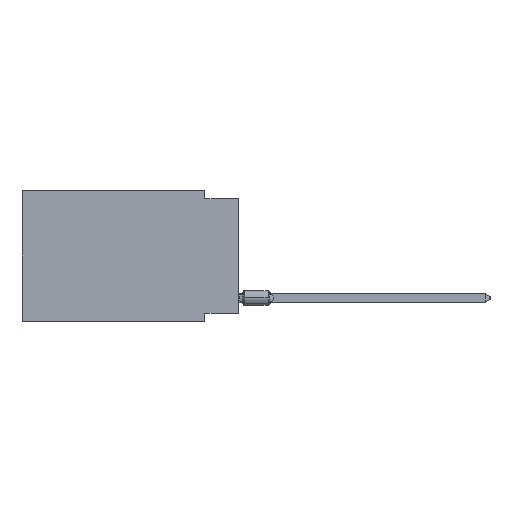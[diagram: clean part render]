
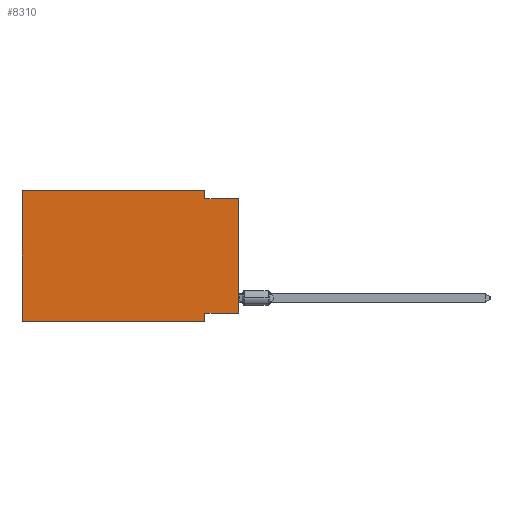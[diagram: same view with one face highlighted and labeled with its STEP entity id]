
A CAD part, left-side view. The second image highlights one B-rep face of the part: STEP entity #8310.
In plain terms, the highlighted planar face has unit normal (-1, 0, 0).
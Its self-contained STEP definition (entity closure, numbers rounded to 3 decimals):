
#1248 = VERTEX_POINT ( 'NONE', #43482 ) ;
#1774 = CARTESIAN_POINT ( 'NONE',  ( 0., 2.54, -9.906 ) ) ;
#2339 = ORIENTED_EDGE ( 'NONE', *, *, #16245, .F. ) ;
#3363 = EDGE_CURVE ( 'NONE', #26355, #38765, #23851, .T. ) ;
#3479 = VECTOR ( 'NONE', #33038, 1000. ) ;
#4649 = CARTESIAN_POINT ( 'NONE',  ( 0., 16.383, 0. ) ) ;
#5287 = EDGE_CURVE ( 'NONE', #26355, #52239, #14087, .T. ) ;
#5362 = AXIS2_PLACEMENT_3D ( 'NONE', #9798, #10987, #5902 ) ;
#5902 = DIRECTION ( 'NONE',  ( 0., 0., -1. ) ) ;
#6004 = VERTEX_POINT ( 'NONE', #13868 ) ;
#6097 = ORIENTED_EDGE ( 'NONE', *, *, #58985, .F. ) ;
#7154 = EDGE_CURVE ( 'NONE', #30819, #1248, #32797, .T. ) ;
#8310 = ADVANCED_FACE ( 'NONE', ( #32629 ), #10387, .F. ) ;
#9240 = VERTEX_POINT ( 'NONE', #26784 ) ;
#9586 = ORIENTED_EDGE ( 'NONE', *, *, #5287, .T. ) ;
#9798 = CARTESIAN_POINT ( 'NONE',  ( 0., 16.383, 0. ) ) ;
#10387 = PLANE ( 'NONE',  #5362 ) ;
#10987 = DIRECTION ( 'NONE',  ( 1., 0., 0. ) ) ;
#11818 = DIRECTION ( 'NONE',  ( 0., 1., 0. ) ) ;
#13607 = VECTOR ( 'NONE', #55955, 1000. ) ;
#13868 = CARTESIAN_POINT ( 'NONE',  ( 0., 2.54, 0. ) ) ;
#14087 = LINE ( 'NONE', #14392, #50177 ) ;
#14392 = CARTESIAN_POINT ( 'NONE',  ( 0., 16.383, -9.906 ) ) ;
#15633 = LINE ( 'NONE', #28853, #33295 ) ;
#16245 = EDGE_CURVE ( 'NONE', #48745, #52239, #25973, .T. ) ;
#20463 = VECTOR ( 'NONE', #31379, 1000. ) ;
#20588 = DIRECTION ( 'NONE',  ( 0., 0., -1. ) ) ;
#21037 = EDGE_CURVE ( 'NONE', #38765, #6004, #27648, .T. ) ;
#22013 = LINE ( 'NONE', #44787, #28293 ) ;
#22168 = CARTESIAN_POINT ( 'NONE',  ( 0., 0., -9.271 ) ) ;
#23208 = VECTOR ( 'NONE', #20588, 1000. ) ;
#23851 = LINE ( 'NONE', #4649, #13607 ) ;
#25973 = LINE ( 'NONE', #34981, #23208 ) ;
#26355 = VERTEX_POINT ( 'NONE', #35169 ) ;
#26784 = CARTESIAN_POINT ( 'NONE',  ( 0., 2.54, -0.635 ) ) ;
#27648 = LINE ( 'NONE', #41142, #3479 ) ;
#28293 = VECTOR ( 'NONE', #11818, 1000. ) ;
#28512 = DIRECTION ( 'NONE',  ( 0., -1., 0. ) ) ;
#28853 = CARTESIAN_POINT ( 'NONE',  ( 0., 0., -0.635 ) ) ;
#29060 = DIRECTION ( 'NONE',  ( 0., 0., -1. ) ) ;
#29637 = CARTESIAN_POINT ( 'NONE',  ( 0., 2.54, 0. ) ) ;
#29727 = EDGE_CURVE ( 'NONE', #6004, #9240, #52434, .T. ) ;
#30819 = VERTEX_POINT ( 'NONE', #22168 ) ;
#31379 = DIRECTION ( 'NONE',  ( 0., 0., 1. ) ) ;
#32629 = FACE_OUTER_BOUND ( 'NONE', #50534, .T. ) ;
#32797 = LINE ( 'NONE', #37291, #20463 ) ;
#33038 = DIRECTION ( 'NONE',  ( 0., -1., 0. ) ) ;
#33295 = VECTOR ( 'NONE', #56135, 1000. ) ;
#34981 = CARTESIAN_POINT ( 'NONE',  ( 0., 2.54, -9.906 ) ) ;
#35169 = CARTESIAN_POINT ( 'NONE',  ( 0., 16.383, -9.906 ) ) ;
#37291 = CARTESIAN_POINT ( 'NONE',  ( 0., 0., 0. ) ) ;
#38765 = VERTEX_POINT ( 'NONE', #40150 ) ;
#40149 = ORIENTED_EDGE ( 'NONE', *, *, #29727, .F. ) ;
#40150 = CARTESIAN_POINT ( 'NONE',  ( 0., 16.383, 0. ) ) ;
#41142 = CARTESIAN_POINT ( 'NONE',  ( 0., 16.383, 0. ) ) ;
#41267 = ORIENTED_EDGE ( 'NONE', *, *, #7154, .T. ) ;
#43018 = ORIENTED_EDGE ( 'NONE', *, *, #21037, .F. ) ;
#43482 = CARTESIAN_POINT ( 'NONE',  ( 0., 0., -0.635 ) ) ;
#44787 = CARTESIAN_POINT ( 'NONE',  ( 0., 0., -9.271 ) ) ;
#48745 = VERTEX_POINT ( 'NONE', #52466 ) ;
#50177 = VECTOR ( 'NONE', #28512, 1000. ) ;
#50366 = ORIENTED_EDGE ( 'NONE', *, *, #3363, .F. ) ;
#50534 = EDGE_LOOP ( 'NONE', ( #41267, #6097, #40149, #43018, #50366, #9586, #2339, #52209 ) ) ;
#52209 = ORIENTED_EDGE ( 'NONE', *, *, #55798, .F. ) ;
#52239 = VERTEX_POINT ( 'NONE', #1774 ) ;
#52434 = LINE ( 'NONE', #29637, #57898 ) ;
#52466 = CARTESIAN_POINT ( 'NONE',  ( 0., 2.54, -9.271 ) ) ;
#55798 = EDGE_CURVE ( 'NONE', #30819, #48745, #22013, .T. ) ;
#55955 = DIRECTION ( 'NONE',  ( 0., 0., 1. ) ) ;
#56135 = DIRECTION ( 'NONE',  ( 0., -1., 0. ) ) ;
#57898 = VECTOR ( 'NONE', #29060, 1000. ) ;
#58985 = EDGE_CURVE ( 'NONE', #9240, #1248, #15633, .T. ) ;
